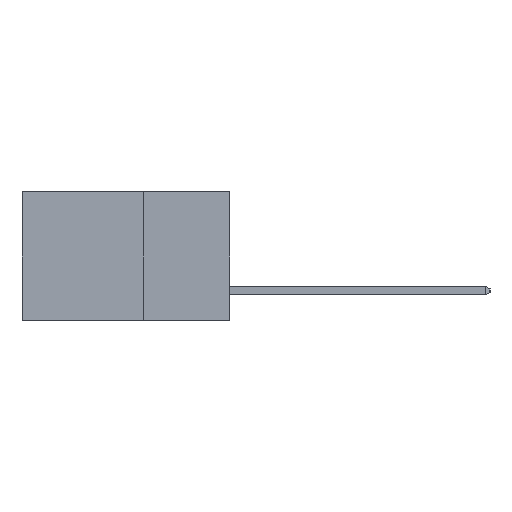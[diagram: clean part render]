
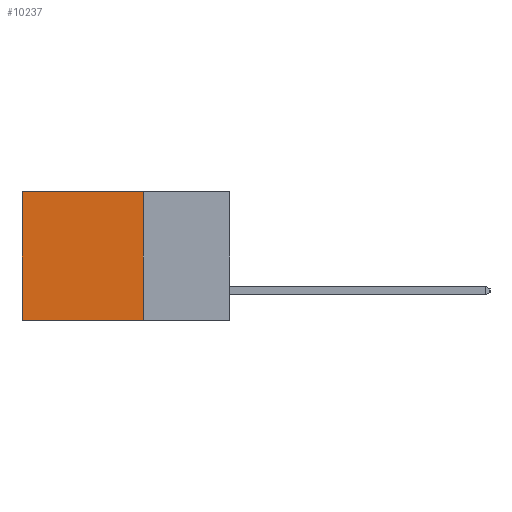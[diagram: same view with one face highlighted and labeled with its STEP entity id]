
A CAD part, left-side view. The second image highlights one B-rep face of the part: STEP entity #10237.
In plain terms, the highlighted planar face has unit normal (-1, 0, 0).
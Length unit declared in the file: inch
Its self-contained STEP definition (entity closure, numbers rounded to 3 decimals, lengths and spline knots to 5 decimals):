
#657 = LINE ( 'NONE', #9342, #3762 ) ;
#1419 = CARTESIAN_POINT ( 'NONE',  ( 0.2615, 0.6, -0.37 ) ) ;
#1469 = DIRECTION ( 'NONE',  ( 0., 0., -1. ) ) ;
#1622 = CARTESIAN_POINT ( 'NONE',  ( 0.2615, 0.25, 0. ) ) ;
#1764 = VERTEX_POINT ( 'NONE', #11944 ) ;
#2155 = LINE ( 'NONE', #1419, #6776 ) ;
#2206 = EDGE_CURVE ( 'NONE', #8228, #1764, #2155, .T. ) ;
#2304 = VERTEX_POINT ( 'NONE', #1622 ) ;
#2519 = EDGE_CURVE ( 'NONE', #2304, #4516, #13489, .T. ) ;
#2530 = VECTOR ( 'NONE', #3880, 39.37008 ) ;
#2825 = ORIENTED_EDGE ( 'NONE', *, *, #5034, .T. ) ;
#3195 = DIRECTION ( 'NONE',  ( 0., 1., 0. ) ) ;
#3434 = CARTESIAN_POINT ( 'NONE',  ( 0.2615, 0.25, -0.37 ) ) ;
#3445 = EDGE_CURVE ( 'NONE', #4516, #1764, #657, .T. ) ;
#3762 = VECTOR ( 'NONE', #9446, 39.37008 ) ;
#3852 = FACE_OUTER_BOUND ( 'NONE', #9310, .T. ) ;
#3880 = DIRECTION ( 'NONE',  ( 0., 0., -1. ) ) ;
#3959 = ORIENTED_EDGE ( 'NONE', *, *, #2519, .F. ) ;
#3987 = CARTESIAN_POINT ( 'NONE',  ( 0.2615, 0.25, -0.37 ) ) ;
#4516 = VERTEX_POINT ( 'NONE', #10372 ) ;
#5034 = EDGE_CURVE ( 'NONE', #2304, #8228, #12833, .T. ) ;
#5644 = DIRECTION ( 'NONE',  ( 1., 0., 0. ) ) ;
#5702 = CARTESIAN_POINT ( 'NONE',  ( 0.2615, 0.25, 0. ) ) ;
#6503 = AXIS2_PLACEMENT_3D ( 'NONE', #3434, #5644, #13986 ) ;
#6776 = VECTOR ( 'NONE', #1469, 39.37008 ) ;
#7962 = ORIENTED_EDGE ( 'NONE', *, *, #3445, .F. ) ;
#8228 = VERTEX_POINT ( 'NONE', #9980 ) ;
#9310 = EDGE_LOOP ( 'NONE', ( #12413, #7962, #3959, #2825 ) ) ;
#9342 = CARTESIAN_POINT ( 'NONE',  ( 0.2615, 0.25, -0.37 ) ) ;
#9446 = DIRECTION ( 'NONE',  ( 0., 1., 0. ) ) ;
#9980 = CARTESIAN_POINT ( 'NONE',  ( 0.2615, 0.6, 0. ) ) ;
#10237 = ADVANCED_FACE ( 'NONE', ( #3852 ), #14135, .F. ) ;
#10372 = CARTESIAN_POINT ( 'NONE',  ( 0.2615, 0.25, -0.37 ) ) ;
#11332 = VECTOR ( 'NONE', #3195, 39.37008 ) ;
#11944 = CARTESIAN_POINT ( 'NONE',  ( 0.2615, 0.6, -0.37 ) ) ;
#12413 = ORIENTED_EDGE ( 'NONE', *, *, #2206, .T. ) ;
#12833 = LINE ( 'NONE', #5702, #11332 ) ;
#13489 = LINE ( 'NONE', #3987, #2530 ) ;
#13986 = DIRECTION ( 'NONE',  ( 0., 0., -1. ) ) ;
#14135 = PLANE ( 'NONE',  #6503 ) ;
